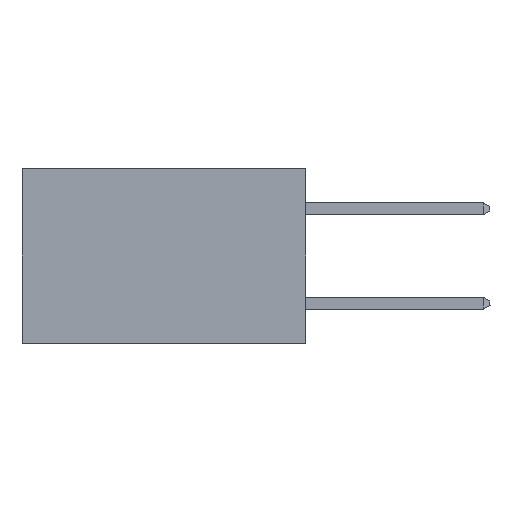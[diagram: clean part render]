
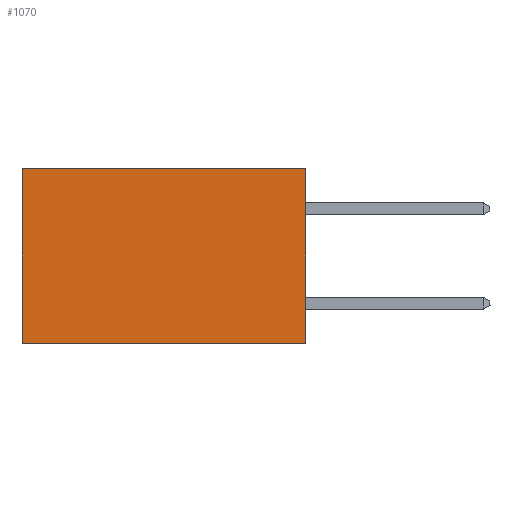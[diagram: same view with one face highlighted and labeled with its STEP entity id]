
A CAD part, left-side view. The second image highlights one B-rep face of the part: STEP entity #1070.
In plain terms, the highlighted planar face has unit normal (-1, 0, 0).
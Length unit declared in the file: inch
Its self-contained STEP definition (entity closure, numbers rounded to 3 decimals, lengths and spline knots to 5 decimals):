
#759 = VERTEX_POINT ( 'NONE', #10553 ) ;
#1070 = ADVANCED_FACE ( 'NONE', ( #18156 ), #22481, .F. ) ;
#1379 = ORIENTED_EDGE ( 'NONE', *, *, #20202, .T. ) ;
#1867 = VERTEX_POINT ( 'NONE', #22169 ) ;
#1900 = CARTESIAN_POINT ( 'NONE',  ( 0.298, 0., 0. ) ) ;
#2162 = DIRECTION ( 'NONE',  ( 0., 0., -1. ) ) ;
#2229 = VECTOR ( 'NONE', #2162, 39.37008 ) ;
#2957 = DIRECTION ( 'NONE',  ( 1., 0., 0. ) ) ;
#3934 = DIRECTION ( 'NONE',  ( 0., 0., -1. ) ) ;
#4532 = CARTESIAN_POINT ( 'NONE',  ( 0.298, 0., -0.37 ) ) ;
#4801 = VECTOR ( 'NONE', #8813, 39.37008 ) ;
#5801 = ORIENTED_EDGE ( 'NONE', *, *, #24215, .T. ) ;
#8813 = DIRECTION ( 'NONE',  ( 0., 1., 0. ) ) ;
#9364 = EDGE_CURVE ( 'NONE', #22931, #10497, #10626, .T. ) ;
#9611 = CARTESIAN_POINT ( 'NONE',  ( 0.298, 0., -0.37 ) ) ;
#10389 = ORIENTED_EDGE ( 'NONE', *, *, #16185, .F. ) ;
#10497 = VERTEX_POINT ( 'NONE', #11864 ) ;
#10553 = CARTESIAN_POINT ( 'NONE',  ( 0.298, 0., 0. ) ) ;
#10626 = LINE ( 'NONE', #9611, #4801 ) ;
#11629 = VECTOR ( 'NONE', #23189, 39.37008 ) ;
#11859 = CARTESIAN_POINT ( 'NONE',  ( 0.298, 0., 0. ) ) ;
#11864 = CARTESIAN_POINT ( 'NONE',  ( 0.298, 0.6, -0.37 ) ) ;
#11942 = CARTESIAN_POINT ( 'NONE',  ( 0.298, 0.6, 0. ) ) ;
#12222 = LINE ( 'NONE', #21413, #11629 ) ;
#13830 = LINE ( 'NONE', #11942, #2229 ) ;
#16185 = EDGE_CURVE ( 'NONE', #759, #22931, #18818, .T. ) ;
#18149 = AXIS2_PLACEMENT_3D ( 'NONE', #11859, #2957, #23222 ) ;
#18156 = FACE_OUTER_BOUND ( 'NONE', #23076, .T. ) ;
#18221 = VECTOR ( 'NONE', #3934, 39.37008 ) ;
#18818 = LINE ( 'NONE', #1900, #18221 ) ;
#19500 = ORIENTED_EDGE ( 'NONE', *, *, #9364, .F. ) ;
#20202 = EDGE_CURVE ( 'NONE', #759, #1867, #12222, .T. ) ;
#21413 = CARTESIAN_POINT ( 'NONE',  ( 0.298, 0., 0. ) ) ;
#22169 = CARTESIAN_POINT ( 'NONE',  ( 0.298, 0.6, 0. ) ) ;
#22481 = PLANE ( 'NONE',  #18149 ) ;
#22931 = VERTEX_POINT ( 'NONE', #4532 ) ;
#23076 = EDGE_LOOP ( 'NONE', ( #5801, #19500, #10389, #1379 ) ) ;
#23189 = DIRECTION ( 'NONE',  ( 0., 1., 0. ) ) ;
#23222 = DIRECTION ( 'NONE',  ( 0., 0., -1. ) ) ;
#24215 = EDGE_CURVE ( 'NONE', #1867, #10497, #13830, .T. ) ;
